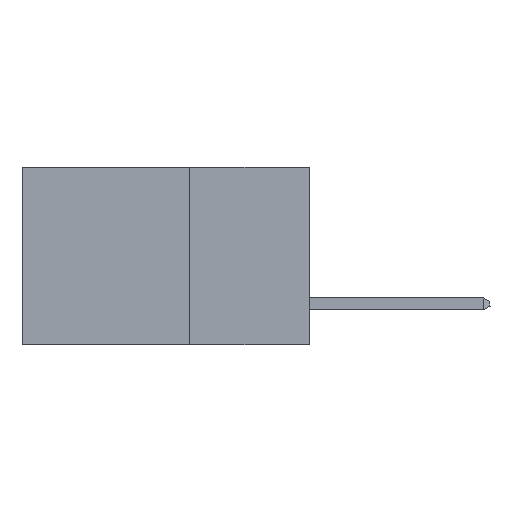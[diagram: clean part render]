
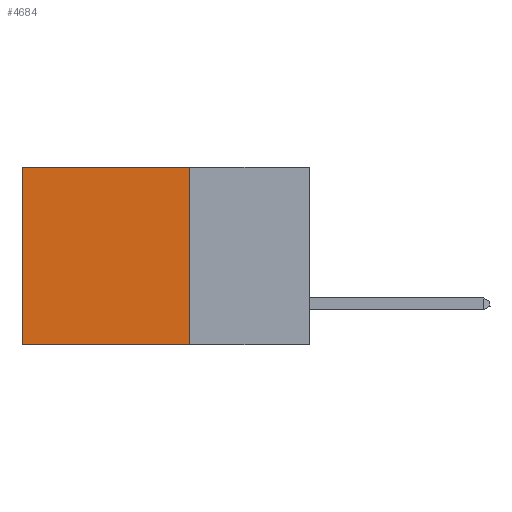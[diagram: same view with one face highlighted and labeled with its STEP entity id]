
A CAD part, left-side view. The second image highlights one B-rep face of the part: STEP entity #4684.
In plain terms, the highlighted planar face has unit normal (-1, 0, 0).
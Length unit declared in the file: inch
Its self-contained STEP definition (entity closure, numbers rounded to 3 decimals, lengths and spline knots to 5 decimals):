
#2423 = AXIS2_PLACEMENT_3D ( 'NONE', #26630, #29016, #23765 ) ;
#2567 = VERTEX_POINT ( 'NONE', #34943 ) ;
#3895 = VERTEX_POINT ( 'NONE', #13113 ) ;
#3955 = EDGE_CURVE ( 'NONE', #3895, #31188, #20667, .T. ) ;
#4684 = ADVANCED_FACE ( 'NONE', ( #28292 ), #13125, .F. ) ;
#5108 = CARTESIAN_POINT ( 'NONE',  ( 0.2875, 0.25, -0.37 ) ) ;
#5526 = DIRECTION ( 'NONE',  ( 0., 1., 0. ) ) ;
#6413 = DIRECTION ( 'NONE',  ( 0., 0., -1. ) ) ;
#7032 = EDGE_CURVE ( 'NONE', #2567, #32294, #7564, .T. ) ;
#7564 = LINE ( 'NONE', #17309, #33094 ) ;
#8425 = EDGE_LOOP ( 'NONE', ( #21570, #10023, #20803, #32890 ) ) ;
#10023 = ORIENTED_EDGE ( 'NONE', *, *, #21543, .F. ) ;
#11409 = CARTESIAN_POINT ( 'NONE',  ( 0.2875, 0.25, 0. ) ) ;
#11787 = CARTESIAN_POINT ( 'NONE',  ( 0.2875, 0.6, 0. ) ) ;
#13113 = CARTESIAN_POINT ( 'NONE',  ( 0.2875, 0.6, 0. ) ) ;
#13125 = PLANE ( 'NONE',  #2423 ) ;
#17309 = CARTESIAN_POINT ( 'NONE',  ( 0.2875, 0.25, 0. ) ) ;
#20667 = LINE ( 'NONE', #11787, #27103 ) ;
#20803 = ORIENTED_EDGE ( 'NONE', *, *, #7032, .F. ) ;
#21543 = EDGE_CURVE ( 'NONE', #32294, #31188, #21565, .T. ) ;
#21565 = LINE ( 'NONE', #29524, #26264 ) ;
#21570 = ORIENTED_EDGE ( 'NONE', *, *, #3955, .T. ) ;
#22680 = DIRECTION ( 'NONE',  ( 0., 1., 0. ) ) ;
#23385 = EDGE_CURVE ( 'NONE', #2567, #3895, #34188, .T. ) ;
#23765 = DIRECTION ( 'NONE',  ( 0., 0., -1. ) ) ;
#26264 = VECTOR ( 'NONE', #5526, 39.37008 ) ;
#26630 = CARTESIAN_POINT ( 'NONE',  ( 0.2875, 0.25, 0. ) ) ;
#27013 = VECTOR ( 'NONE', #22680, 39.37008 ) ;
#27103 = VECTOR ( 'NONE', #31020, 39.37008 ) ;
#28292 = FACE_OUTER_BOUND ( 'NONE', #8425, .T. ) ;
#29016 = DIRECTION ( 'NONE',  ( 1., 0., 0. ) ) ;
#29524 = CARTESIAN_POINT ( 'NONE',  ( 0.2875, 0.25, -0.37 ) ) ;
#31020 = DIRECTION ( 'NONE',  ( 0., 0., -1. ) ) ;
#31188 = VERTEX_POINT ( 'NONE', #32937 ) ;
#32294 = VERTEX_POINT ( 'NONE', #5108 ) ;
#32890 = ORIENTED_EDGE ( 'NONE', *, *, #23385, .T. ) ;
#32937 = CARTESIAN_POINT ( 'NONE',  ( 0.2875, 0.6, -0.37 ) ) ;
#33094 = VECTOR ( 'NONE', #6413, 39.37008 ) ;
#34188 = LINE ( 'NONE', #11409, #27013 ) ;
#34943 = CARTESIAN_POINT ( 'NONE',  ( 0.2875, 0.25, 0. ) ) ;
